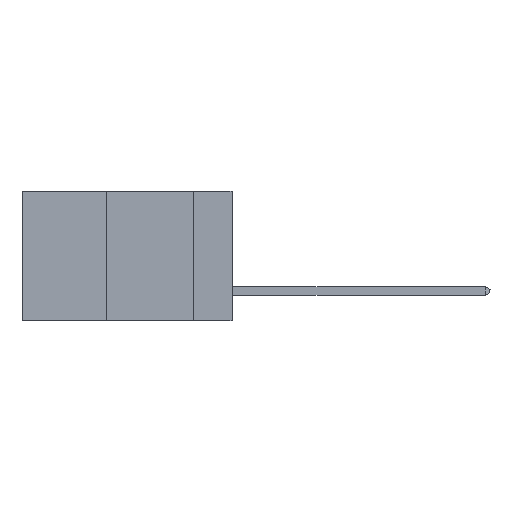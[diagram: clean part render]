
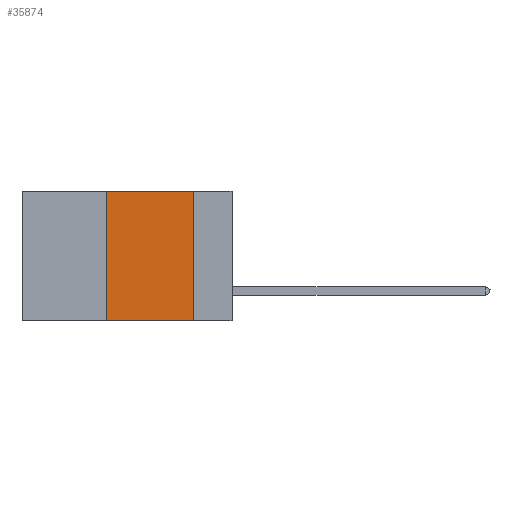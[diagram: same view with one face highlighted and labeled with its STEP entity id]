
A CAD part, left-side view. The second image highlights one B-rep face of the part: STEP entity #35874.
In plain terms, the highlighted planar face has unit normal (-1, 0, 0).
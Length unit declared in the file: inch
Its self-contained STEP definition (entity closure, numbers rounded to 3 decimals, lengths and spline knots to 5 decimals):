
#1667 = CARTESIAN_POINT ( 'NONE',  ( 0., 0.6, 0. ) ) ;
#1704 = EDGE_CURVE ( 'NONE', #5628, #16710, #17061, .T. ) ;
#2236 = CARTESIAN_POINT ( 'NONE',  ( 0., 0.11, -0.37 ) ) ;
#2650 = FACE_OUTER_BOUND ( 'NONE', #12753, .T. ) ;
#3754 = LINE ( 'NONE', #10555, #17892 ) ;
#4624 = CARTESIAN_POINT ( 'NONE',  ( 0., 0.36, 0. ) ) ;
#4904 = ORIENTED_EDGE ( 'NONE', *, *, #29761, .F. ) ;
#5628 = VERTEX_POINT ( 'NONE', #21556 ) ;
#5966 = CARTESIAN_POINT ( 'NONE',  ( 0., 0.6, 0. ) ) ;
#6321 = EDGE_CURVE ( 'NONE', #5628, #6476, #24759, .T. ) ;
#6476 = VERTEX_POINT ( 'NONE', #4624 ) ;
#9038 = DIRECTION ( 'NONE',  ( 0., 0., 1. ) ) ;
#9176 = AXIS2_PLACEMENT_3D ( 'NONE', #5966, #14523, #26482 ) ;
#10555 = CARTESIAN_POINT ( 'NONE',  ( 0., 0.11, 0. ) ) ;
#11563 = EDGE_CURVE ( 'NONE', #34970, #16710, #3754, .T. ) ;
#11899 = PLANE ( 'NONE',  #9176 ) ;
#12753 = EDGE_LOOP ( 'NONE', ( #34757, #4904, #34748, #24456 ) ) ;
#13058 = CARTESIAN_POINT ( 'NONE',  ( 0., 0.6, -0.37 ) ) ;
#14523 = DIRECTION ( 'NONE',  ( 1., 0., 0. ) ) ;
#16151 = VECTOR ( 'NONE', #36816, 39.37008 ) ;
#16710 = VERTEX_POINT ( 'NONE', #2236 ) ;
#17021 = VECTOR ( 'NONE', #9038, 39.37008 ) ;
#17061 = LINE ( 'NONE', #13058, #16151 ) ;
#17892 = VECTOR ( 'NONE', #33975, 39.37008 ) ;
#18627 = CARTESIAN_POINT ( 'NONE',  ( 0., 0.11, 0. ) ) ;
#21556 = CARTESIAN_POINT ( 'NONE',  ( 0., 0.36, -0.37 ) ) ;
#22111 = VECTOR ( 'NONE', #37207, 39.37008 ) ;
#24456 = ORIENTED_EDGE ( 'NONE', *, *, #1704, .T. ) ;
#24759 = LINE ( 'NONE', #26506, #17021 ) ;
#26482 = DIRECTION ( 'NONE',  ( 0., 0., -1. ) ) ;
#26506 = CARTESIAN_POINT ( 'NONE',  ( 0., 0.36, 0. ) ) ;
#29761 = EDGE_CURVE ( 'NONE', #6476, #34970, #35837, .T. ) ;
#33975 = DIRECTION ( 'NONE',  ( 0., 0., -1. ) ) ;
#34748 = ORIENTED_EDGE ( 'NONE', *, *, #6321, .F. ) ;
#34757 = ORIENTED_EDGE ( 'NONE', *, *, #11563, .F. ) ;
#34970 = VERTEX_POINT ( 'NONE', #18627 ) ;
#35837 = LINE ( 'NONE', #1667, #22111 ) ;
#35874 = ADVANCED_FACE ( 'NONE', ( #2650 ), #11899, .F. ) ;
#36816 = DIRECTION ( 'NONE',  ( 0., -1., 0. ) ) ;
#37207 = DIRECTION ( 'NONE',  ( 0., -1., 0. ) ) ;
